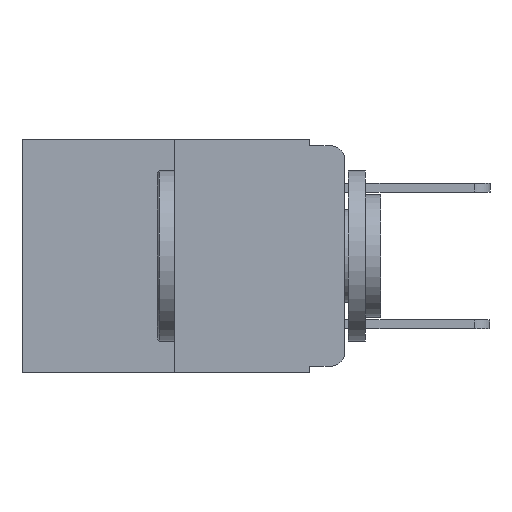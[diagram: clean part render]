
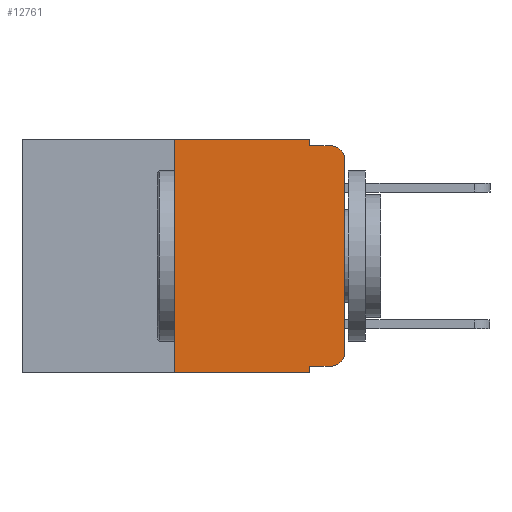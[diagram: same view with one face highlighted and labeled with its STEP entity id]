
A CAD part, left-side view. The second image highlights one B-rep face of the part: STEP entity #12761.
In plain terms, the highlighted planar face has unit normal (-1, 0, 0).
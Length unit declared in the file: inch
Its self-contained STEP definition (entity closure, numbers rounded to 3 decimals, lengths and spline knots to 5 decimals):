
#609 = VERTEX_POINT ( 'NONE', #6191 ) ;
#799 = LINE ( 'NONE', #17018, #8157 ) ;
#944 = CARTESIAN_POINT ( 'NONE',  ( 0., 0., 0. ) ) ;
#1394 = DIRECTION ( 'NONE',  ( 0., 0., -1. ) ) ;
#1577 = CARTESIAN_POINT ( 'NONE',  ( 0., 0.02, -0.01 ) ) ;
#1624 = CARTESIAN_POINT ( 'NONE',  ( 0., 0.051, 0. ) ) ;
#1757 = CARTESIAN_POINT ( 'NONE',  ( 0., 0.25, 0. ) ) ;
#1808 = CIRCLE ( 'NONE', #8932, 0.02 ) ;
#2445 = DIRECTION ( 'NONE',  ( 0., -1., 0. ) ) ;
#3071 = VERTEX_POINT ( 'NONE', #3623 ) ;
#3080 = EDGE_CURVE ( 'NONE', #7896, #12660, #8657, .T. ) ;
#3513 = DIRECTION ( 'NONE',  ( 0., -1., 0. ) ) ;
#3623 = CARTESIAN_POINT ( 'NONE',  ( 0., 0.02, -0.333 ) ) ;
#4042 = EDGE_CURVE ( 'NONE', #17731, #7225, #5383, .T. ) ;
#4139 = CARTESIAN_POINT ( 'NONE',  ( 0., 0.051, 0. ) ) ;
#4188 = DIRECTION ( 'NONE',  ( 0., 0., 1. ) ) ;
#4328 = DIRECTION ( 'NONE',  ( 0., 0., -1. ) ) ;
#4427 = EDGE_CURVE ( 'NONE', #609, #12636, #6522, .T. ) ;
#4450 = EDGE_CURVE ( 'NONE', #12636, #4522, #1808, .T. ) ;
#4456 = EDGE_CURVE ( 'NONE', #10497, #4522, #16082, .T. ) ;
#4508 = EDGE_CURVE ( 'NONE', #12660, #10497, #5113, .T. ) ;
#4514 = EDGE_CURVE ( 'NONE', #17731, #7896, #799, .T. ) ;
#4518 = EDGE_CURVE ( 'NONE', #9560, #7225, #4580, .T. ) ;
#4522 = VERTEX_POINT ( 'NONE', #1577 ) ;
#4549 = EDGE_CURVE ( 'NONE', #9560, #3071, #11092, .T. ) ;
#4574 = EDGE_CURVE ( 'NONE', #3071, #609, #11534, .T. ) ;
#4580 = LINE ( 'NONE', #4139, #11922 ) ;
#4698 = DIRECTION ( 'NONE',  ( -1., 0., 0. ) ) ;
#4727 = CARTESIAN_POINT ( 'NONE',  ( 0., 0.02, -0.313 ) ) ;
#4889 = VECTOR ( 'NONE', #8555, 39.37008 ) ;
#5040 = DIRECTION ( 'NONE',  ( 0., 0., -1. ) ) ;
#5113 = LINE ( 'NONE', #1624, #8617 ) ;
#5383 = LINE ( 'NONE', #17216, #4889 ) ;
#5894 = CARTESIAN_POINT ( 'NONE',  ( 0., 0.02, -0.03 ) ) ;
#6073 = VECTOR ( 'NONE', #12134, 39.37008 ) ;
#6086 = CARTESIAN_POINT ( 'NONE',  ( 0., 0.051, -0.343 ) ) ;
#6191 = CARTESIAN_POINT ( 'NONE',  ( 0., 0., -0.313 ) ) ;
#6522 = LINE ( 'NONE', #944, #6073 ) ;
#6550 = EDGE_LOOP ( 'NONE', ( #7919, #8082, #8182, #8241, #8278, #8413, #8441, #8519, #8704, #9094 ) ) ;
#6556 = DIRECTION ( 'NONE',  ( 0., -1., 0. ) ) ;
#6572 = CARTESIAN_POINT ( 'NONE',  ( 0., 0.051, 0. ) ) ;
#6589 = CARTESIAN_POINT ( 'NONE',  ( 0., 0.051, -0.01 ) ) ;
#7212 = VECTOR ( 'NONE', #6556, 39.37008 ) ;
#7225 = VERTEX_POINT ( 'NONE', #6086 ) ;
#7896 = VERTEX_POINT ( 'NONE', #1757 ) ;
#7919 = ORIENTED_EDGE ( 'NONE', *, *, #4427, .T. ) ;
#8082 = ORIENTED_EDGE ( 'NONE', *, *, #4450, .T. ) ;
#8157 = VECTOR ( 'NONE', #4188, 39.37008 ) ;
#8182 = ORIENTED_EDGE ( 'NONE', *, *, #4456, .F. ) ;
#8241 = ORIENTED_EDGE ( 'NONE', *, *, #4508, .F. ) ;
#8278 = ORIENTED_EDGE ( 'NONE', *, *, #3080, .F. ) ;
#8413 = ORIENTED_EDGE ( 'NONE', *, *, #4514, .F. ) ;
#8441 = ORIENTED_EDGE ( 'NONE', *, *, #4042, .T. ) ;
#8519 = ORIENTED_EDGE ( 'NONE', *, *, #4518, .F. ) ;
#8555 = DIRECTION ( 'NONE',  ( 0., -1., 0. ) ) ;
#8617 = VECTOR ( 'NONE', #1394, 39.37008 ) ;
#8657 = LINE ( 'NONE', #15110, #11952 ) ;
#8704 = ORIENTED_EDGE ( 'NONE', *, *, #4549, .T. ) ;
#8932 = AXIS2_PLACEMENT_3D ( 'NONE', #5894, #12492, #5040 ) ;
#9094 = ORIENTED_EDGE ( 'NONE', *, *, #4574, .T. ) ;
#9560 = VERTEX_POINT ( 'NONE', #16736 ) ;
#9988 = DIRECTION ( 'NONE',  ( 0., 0., -1. ) ) ;
#10019 = FACE_OUTER_BOUND ( 'NONE', #6550, .T. ) ;
#10363 = AXIS2_PLACEMENT_3D ( 'NONE', #17436, #17481, #9988 ) ;
#10497 = VERTEX_POINT ( 'NONE', #6589 ) ;
#11092 = LINE ( 'NONE', #12566, #7212 ) ;
#11534 = CIRCLE ( 'NONE', #11762, 0.02 ) ;
#11762 = AXIS2_PLACEMENT_3D ( 'NONE', #4727, #4698, #15989 ) ;
#11922 = VECTOR ( 'NONE', #4328, 39.37008 ) ;
#11952 = VECTOR ( 'NONE', #2445, 39.37008 ) ;
#12134 = DIRECTION ( 'NONE',  ( 0., 0., 1. ) ) ;
#12492 = DIRECTION ( 'NONE',  ( -1., 0., 0. ) ) ;
#12566 = CARTESIAN_POINT ( 'NONE',  ( 0., 0.051, -0.333 ) ) ;
#12636 = VERTEX_POINT ( 'NONE', #13582 ) ;
#12660 = VERTEX_POINT ( 'NONE', #6572 ) ;
#12757 = VECTOR ( 'NONE', #3513, 39.37008 ) ;
#12761 = ADVANCED_FACE ( 'NONE', ( #10019 ), #16418, .F. ) ;
#13582 = CARTESIAN_POINT ( 'NONE',  ( 0., 0., -0.03 ) ) ;
#14302 = CARTESIAN_POINT ( 'NONE',  ( 0., 0.25, -0.343 ) ) ;
#15110 = CARTESIAN_POINT ( 'NONE',  ( 0., 0.473, 0. ) ) ;
#15989 = DIRECTION ( 'NONE',  ( 0., 0., -1. ) ) ;
#16082 = LINE ( 'NONE', #16944, #12757 ) ;
#16418 = PLANE ( 'NONE',  #10363 ) ;
#16736 = CARTESIAN_POINT ( 'NONE',  ( 0., 0.051, -0.333 ) ) ;
#16944 = CARTESIAN_POINT ( 'NONE',  ( 0., 0.051, -0.01 ) ) ;
#17018 = CARTESIAN_POINT ( 'NONE',  ( 0., 0.25, 0. ) ) ;
#17216 = CARTESIAN_POINT ( 'NONE',  ( 0., 0.473, -0.343 ) ) ;
#17436 = CARTESIAN_POINT ( 'NONE',  ( 0., 0.473, 0. ) ) ;
#17481 = DIRECTION ( 'NONE',  ( 1., 0., 0. ) ) ;
#17731 = VERTEX_POINT ( 'NONE', #14302 ) ;
